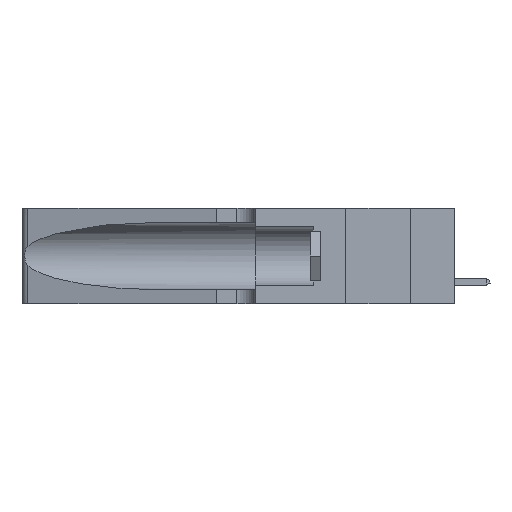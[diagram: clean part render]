
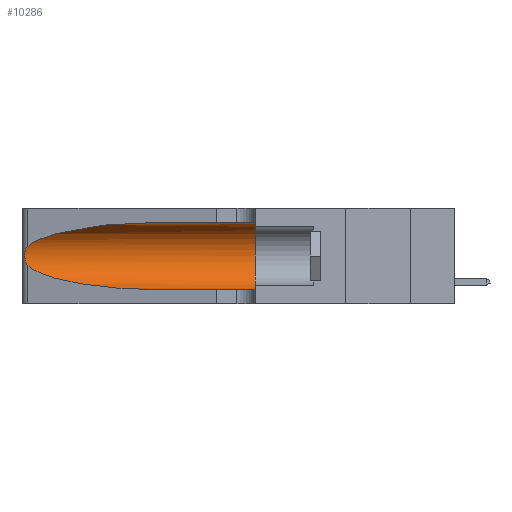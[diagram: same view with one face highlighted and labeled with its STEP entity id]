
A CAD part, left-side view. The second image highlights one B-rep face of the part: STEP entity #10286.
In plain terms, the highlighted cylindrical face has radius 3.308 mm (diameter 6.617 mm), a partial arc.
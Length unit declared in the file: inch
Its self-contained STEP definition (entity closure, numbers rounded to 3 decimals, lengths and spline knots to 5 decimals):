
#111 = B_SPLINE_CURVE_WITH_KNOTS ( 'NONE', 3,
 ( #9239, #30436, #22365, #22246, #22013, #6323, #33023, #32915, #19590, #17091, #6436, #3387, #8988, #32682 ),
 .UNSPECIFIED., .F., .F.,
 ( 4, 2, 2, 2, 2, 2, 4 ),
 ( 0., 0.00027, 0.00053, 0.00107, 0.0016, 0.00187, 0.00214 ),
 .UNSPECIFIED. ) ;
#2230 = CARTESIAN_POINT ( 'NONE',  ( 0.1305, 1.61858, 0.185 ) ) ;
#2828 = AXIS2_PLACEMENT_3D ( 'NONE', #32458, #3180, #16738 ) ;
#3180 = DIRECTION ( 'NONE',  ( 0., 1., 0. ) ) ;
#3278 = CARTESIAN_POINT ( 'NONE',  ( 0.1305, 1.61858, 0.31525 ) ) ;
#3387 = CARTESIAN_POINT ( 'NONE',  ( 0.25639, 1.23186, 0.15144 ) ) ;
#4166 =( BOUNDED_CURVE ( )  B_SPLINE_CURVE ( 3, ( #10294, #29142, #34555, #26321 ),
 .UNSPECIFIED., .F., .T. ) 
 B_SPLINE_CURVE_WITH_KNOTS ( ( 4, 4 ),
 ( 1.5708, 2.84003 ),
 .UNSPECIFIED. ) 
 CURVE ( )  GEOMETRIC_REPRESENTATION_ITEM ( )  RATIONAL_B_SPLINE_CURVE ( ( 1., 0.87, 0.87, 1. ) ) 
 REPRESENTATION_ITEM ( '' )  );
#4273 = VERTEX_POINT ( 'NONE', #8036 ) ;
#5089 = ORIENTED_EDGE ( 'NONE', *, *, #33259, .F. ) ;
#5666 = VECTOR ( 'NONE', #14127, 39.37008 ) ;
#5890 = EDGE_CURVE ( 'NONE', #9670, #4273, #111, .T. ) ;
#6191 = CARTESIAN_POINT ( 'NONE',  ( 0.25487, 1.22718, 0.14631 ) ) ;
#6230 = CARTESIAN_POINT ( 'NONE',  ( 0.1305, 0.72297, 0.31525 ) ) ;
#6323 = CARTESIAN_POINT ( 'NONE',  ( 0.26018, 1.23835, 0.19895 ) ) ;
#6436 = CARTESIAN_POINT ( 'NONE',  ( 0.25789, 1.23486, 0.15765 ) ) ;
#8036 = CARTESIAN_POINT ( 'NONE',  ( 0.25487, 1.22718, 0.14631 ) ) ;
#8988 = CARTESIAN_POINT ( 'NONE',  ( 0.25555, 1.22993, 0.14849 ) ) ;
#9239 = CARTESIAN_POINT ( 'NONE',  ( 0.25487, 1.22718, 0.22369 ) ) ;
#9670 = VERTEX_POINT ( 'NONE', #13295 ) ;
#10286 = ADVANCED_FACE ( 'NONE', ( #19365 ), #12291, .F. ) ;
#10294 = CARTESIAN_POINT ( 'NONE',  ( 0.1305, 0.72297, 0.31525 ) ) ;
#10682 = LINE ( 'NONE', #20043, #22291 ) ;
#11310 = CARTESIAN_POINT ( 'NONE',  ( 0.2373, 1.15595, 0.08982 ) ) ;
#11412 = VERTEX_POINT ( 'NONE', #6230 ) ;
#11835 =( BOUNDED_CURVE ( )  B_SPLINE_CURVE ( 3, ( #6191, #11310, #22125, #29958 ),
 .UNSPECIFIED., .F., .F. ) 
 B_SPLINE_CURVE_WITH_KNOTS ( ( 4, 4 ),
 ( 3.44316, 4.71239 ),
 .UNSPECIFIED. ) 
 CURVE ( )  GEOMETRIC_REPRESENTATION_ITEM ( )  RATIONAL_B_SPLINE_CURVE ( ( 1., 0.87, 0.87, 1. ) ) 
 REPRESENTATION_ITEM ( '' )  );
#12291 = CYLINDRICAL_SURFACE ( 'NONE', #22815, 0.13025 ) ;
#12350 = CARTESIAN_POINT ( 'NONE',  ( 0.1305, 0.35, 0.05475 ) ) ;
#13295 = CARTESIAN_POINT ( 'NONE',  ( 0.25487, 1.22718, 0.22369 ) ) ;
#14127 = DIRECTION ( 'NONE',  ( 0., -1., 0. ) ) ;
#15075 = DIRECTION ( 'NONE',  ( 0., 0., -1. ) ) ;
#16738 = DIRECTION ( 'NONE',  ( 0., 0., 1. ) ) ;
#16982 = ORIENTED_EDGE ( 'NONE', *, *, #5890, .T. ) ;
#17091 = CARTESIAN_POINT ( 'NONE',  ( 0.25856, 1.23593, 0.16098 ) ) ;
#17248 = EDGE_CURVE ( 'NONE', #4273, #22211, #11835, .T. ) ;
#19365 = FACE_OUTER_BOUND ( 'NONE', #23829, .T. ) ;
#19590 = CARTESIAN_POINT ( 'NONE',  ( 0.26017, 1.23833, 0.17102 ) ) ;
#19904 = ORIENTED_EDGE ( 'NONE', *, *, #28405, .F. ) ;
#20043 = CARTESIAN_POINT ( 'NONE',  ( 0.1305, 1.61858, 0.05475 ) ) ;
#20409 = EDGE_CURVE ( 'NONE', #11412, #9670, #4166, .T. ) ;
#20729 = DIRECTION ( 'NONE',  ( 0., -1., 0. ) ) ;
#22013 = CARTESIAN_POINT ( 'NONE',  ( 0.25854, 1.2359, 0.20912 ) ) ;
#22125 = CARTESIAN_POINT ( 'NONE',  ( 0.18966, 0.96281, 0.05475 ) ) ;
#22211 = VERTEX_POINT ( 'NONE', #29357 ) ;
#22246 = CARTESIAN_POINT ( 'NONE',  ( 0.25787, 1.23484, 0.2124 ) ) ;
#22291 = VECTOR ( 'NONE', #30779, 39.37008 ) ;
#22365 = CARTESIAN_POINT ( 'NONE',  ( 0.25639, 1.23184, 0.21858 ) ) ;
#22815 = AXIS2_PLACEMENT_3D ( 'NONE', #2230, #20729, #15075 ) ;
#23829 = EDGE_LOOP ( 'NONE', ( #30261, #16982, #32181, #25908, #5089, #19904 ) ) ;
#25764 = CIRCLE ( 'NONE', #2828, 0.13025 ) ;
#25908 = ORIENTED_EDGE ( 'NONE', *, *, #34158, .T. ) ;
#26321 = CARTESIAN_POINT ( 'NONE',  ( 0.25487, 1.22718, 0.22369 ) ) ;
#28189 = VERTEX_POINT ( 'NONE', #12350 ) ;
#28405 = EDGE_CURVE ( 'NONE', #11412, #30931, #31977, .T. ) ;
#29142 = CARTESIAN_POINT ( 'NONE',  ( 0.18966, 0.96281, 0.31525 ) ) ;
#29357 = CARTESIAN_POINT ( 'NONE',  ( 0.1305, 0.72297, 0.05475 ) ) ;
#29958 = CARTESIAN_POINT ( 'NONE',  ( 0.1305, 0.72297, 0.05475 ) ) ;
#30131 = CARTESIAN_POINT ( 'NONE',  ( 0.1305, 0.35, 0.31525 ) ) ;
#30261 = ORIENTED_EDGE ( 'NONE', *, *, #20409, .T. ) ;
#30436 = CARTESIAN_POINT ( 'NONE',  ( 0.25555, 1.22994, 0.2215 ) ) ;
#30779 = DIRECTION ( 'NONE',  ( 0., -1., 0. ) ) ;
#30931 = VERTEX_POINT ( 'NONE', #30131 ) ;
#31977 = LINE ( 'NONE', #3278, #5666 ) ;
#32181 = ORIENTED_EDGE ( 'NONE', *, *, #17248, .T. ) ;
#32458 = CARTESIAN_POINT ( 'NONE',  ( 0.1305, 0.35, 0.185 ) ) ;
#32682 = CARTESIAN_POINT ( 'NONE',  ( 0.25487, 1.22718, 0.14631 ) ) ;
#32915 = CARTESIAN_POINT ( 'NONE',  ( 0.26075, 1.23896, 0.178 ) ) ;
#33023 = CARTESIAN_POINT ( 'NONE',  ( 0.26075, 1.23896, 0.19203 ) ) ;
#33259 = EDGE_CURVE ( 'NONE', #30931, #28189, #25764, .T. ) ;
#34158 = EDGE_CURVE ( 'NONE', #22211, #28189, #10682, .T. ) ;
#34555 = CARTESIAN_POINT ( 'NONE',  ( 0.2373, 1.15595, 0.28018 ) ) ;
